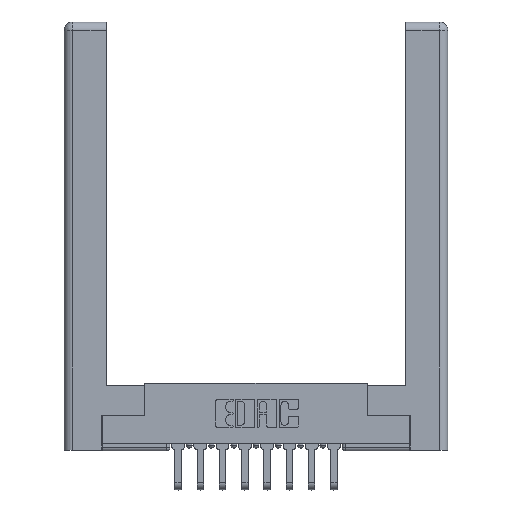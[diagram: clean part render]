
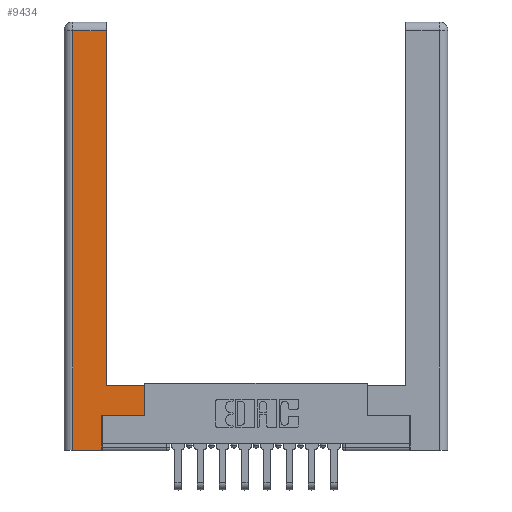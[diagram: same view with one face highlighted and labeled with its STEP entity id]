
A CAD part, top view. The second image highlights one B-rep face of the part: STEP entity #9434.
In plain terms, the highlighted planar face has unit normal (0, 0, 1).
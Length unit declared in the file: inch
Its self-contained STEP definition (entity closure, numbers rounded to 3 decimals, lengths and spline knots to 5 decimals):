
#355 = CARTESIAN_POINT ( 'NONE',  ( 0.295, 0.45, 0. ) ) ;
#687 = CARTESIAN_POINT ( 'NONE',  ( 0.565, 0.245, 0. ) ) ;
#735 = VECTOR ( 'NONE', #8342, 39.37008 ) ;
#1167 = VECTOR ( 'NONE', #3853, 39.37008 ) ;
#1283 = VERTEX_POINT ( 'NONE', #9813 ) ;
#1554 = EDGE_CURVE ( 'NONE', #4206, #11275, #12857, .T. ) ;
#1744 = ORIENTED_EDGE ( 'NONE', *, *, #8564, .T. ) ;
#1896 = EDGE_CURVE ( 'NONE', #2811, #9806, #9670, .T. ) ;
#1959 = VERTEX_POINT ( 'NONE', #4827 ) ;
#2538 = FACE_OUTER_BOUND ( 'NONE', #8995, .T. ) ;
#2691 = CARTESIAN_POINT ( 'NONE',  ( 0.295, 3., 0. ) ) ;
#2811 = VERTEX_POINT ( 'NONE', #3128 ) ;
#2865 = VERTEX_POINT ( 'NONE', #10698 ) ;
#2878 = LINE ( 'NONE', #10606, #735 ) ;
#2882 = ORIENTED_EDGE ( 'NONE', *, *, #1554, .T. ) ;
#2891 = LINE ( 'NONE', #13388, #9242 ) ;
#3128 = CARTESIAN_POINT ( 'NONE',  ( 0.295, 0.45, 0. ) ) ;
#3182 = ORIENTED_EDGE ( 'NONE', *, *, #4706, .T. ) ;
#3540 = VECTOR ( 'NONE', #12881, 39.37008 ) ;
#3774 = DIRECTION ( 'NONE',  ( 0., 1., 0. ) ) ;
#3853 = DIRECTION ( 'NONE',  ( 0., 1., 0. ) ) ;
#4023 = ORIENTED_EDGE ( 'NONE', *, *, #8128, .T. ) ;
#4206 = VERTEX_POINT ( 'NONE', #5898 ) ;
#4706 = EDGE_CURVE ( 'NONE', #1283, #2811, #10927, .T. ) ;
#4758 = EDGE_CURVE ( 'NONE', #9806, #12516, #2891, .T. ) ;
#4827 = CARTESIAN_POINT ( 'NONE',  ( 0.265, 0., 0. ) ) ;
#4974 = DIRECTION ( 'NONE',  ( 1., 0., 0. ) ) ;
#5594 = CARTESIAN_POINT ( 'NONE',  ( 0.565, 0.45, 0. ) ) ;
#5749 = ORIENTED_EDGE ( 'NONE', *, *, #1896, .T. ) ;
#5898 = CARTESIAN_POINT ( 'NONE',  ( 0.265, 0.245, 0. ) ) ;
#6264 = VECTOR ( 'NONE', #4974, 39.37008 ) ;
#6265 = CARTESIAN_POINT ( 'NONE',  ( 0.0615, 2.94, 0. ) ) ;
#7727 = ORIENTED_EDGE ( 'NONE', *, *, #13756, .T. ) ;
#7754 = EDGE_CURVE ( 'NONE', #12516, #2865, #2878, .T. ) ;
#7907 = LINE ( 'NONE', #13434, #6264 ) ;
#8128 = EDGE_CURVE ( 'NONE', #1959, #4206, #12753, .T. ) ;
#8342 = DIRECTION ( 'NONE',  ( 0., -1., 0. ) ) ;
#8375 = DIRECTION ( 'NONE',  ( 1., 0., 0. ) ) ;
#8564 = EDGE_CURVE ( 'NONE', #11275, #1283, #8875, .T. ) ;
#8875 = LINE ( 'NONE', #5594, #3540 ) ;
#8889 = VECTOR ( 'NONE', #11026, 39.37008 ) ;
#8995 = EDGE_LOOP ( 'NONE', ( #5749, #9556, #13685, #7727, #4023, #2882, #1744, #3182 ) ) ;
#9242 = VECTOR ( 'NONE', #10055, 39.37008 ) ;
#9434 = ADVANCED_FACE ( 'NONE', ( #2538 ), #11425, .F. ) ;
#9456 = AXIS2_PLACEMENT_3D ( 'NONE', #10383, #11282, #13457 ) ;
#9556 = ORIENTED_EDGE ( 'NONE', *, *, #4758, .T. ) ;
#9670 = LINE ( 'NONE', #2691, #1167 ) ;
#9806 = VERTEX_POINT ( 'NONE', #11822 ) ;
#9813 = CARTESIAN_POINT ( 'NONE',  ( 0.565, 0.45, 0. ) ) ;
#9926 = VECTOR ( 'NONE', #3774, 39.37008 ) ;
#10025 = VECTOR ( 'NONE', #8375, 39.37008 ) ;
#10055 = DIRECTION ( 'NONE',  ( -1., 0., 0. ) ) ;
#10383 = CARTESIAN_POINT ( 'NONE',  ( 0., 0., 0. ) ) ;
#10606 = CARTESIAN_POINT ( 'NONE',  ( 0.0615, 0., 0. ) ) ;
#10698 = CARTESIAN_POINT ( 'NONE',  ( 0.0615, 0., 0. ) ) ;
#10927 = LINE ( 'NONE', #355, #8889 ) ;
#11026 = DIRECTION ( 'NONE',  ( -1., 0., 0. ) ) ;
#11275 = VERTEX_POINT ( 'NONE', #687 ) ;
#11282 = DIRECTION ( 'NONE',  ( 0., 0., -1. ) ) ;
#11425 = PLANE ( 'NONE',  #9456 ) ;
#11822 = CARTESIAN_POINT ( 'NONE',  ( 0.295, 2.94, 0. ) ) ;
#12516 = VERTEX_POINT ( 'NONE', #6265 ) ;
#12744 = CARTESIAN_POINT ( 'NONE',  ( 0.565, 0.245, 0. ) ) ;
#12753 = LINE ( 'NONE', #13444, #9926 ) ;
#12857 = LINE ( 'NONE', #12744, #10025 ) ;
#12881 = DIRECTION ( 'NONE',  ( 0., 1., 0. ) ) ;
#13388 = CARTESIAN_POINT ( 'NONE',  ( 0.0615, 2.94, 0. ) ) ;
#13434 = CARTESIAN_POINT ( 'NONE',  ( 0.265, 0., 0. ) ) ;
#13444 = CARTESIAN_POINT ( 'NONE',  ( 0.265, 0.245, 0. ) ) ;
#13457 = DIRECTION ( 'NONE',  ( -1., 0., 0. ) ) ;
#13685 = ORIENTED_EDGE ( 'NONE', *, *, #7754, .T. ) ;
#13756 = EDGE_CURVE ( 'NONE', #2865, #1959, #7907, .T. ) ;
